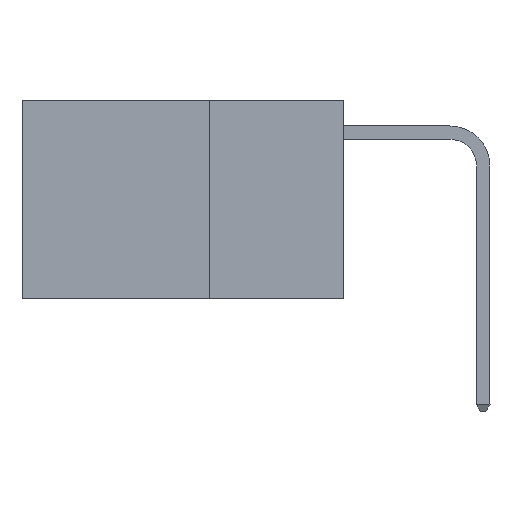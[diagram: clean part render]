
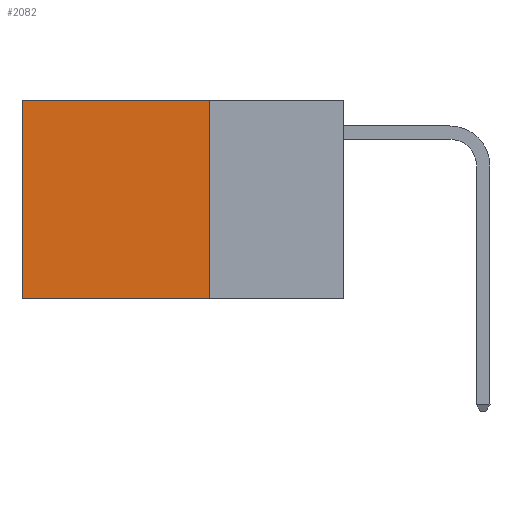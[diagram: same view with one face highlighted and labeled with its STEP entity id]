
A CAD part, left-side view. The second image highlights one B-rep face of the part: STEP entity #2082.
In plain terms, the highlighted planar face has unit normal (-1, 0, 0).
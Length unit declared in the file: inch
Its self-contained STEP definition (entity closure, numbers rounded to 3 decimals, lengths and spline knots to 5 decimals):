
#605 = VERTEX_POINT ( 'NONE', #11744 ) ;
#836 = LINE ( 'NONE', #6273, #850 ) ;
#850 = VECTOR ( 'NONE', #6244, 39.37008 ) ;
#907 = DIRECTION ( 'NONE',  ( 0., 0., -1. ) ) ;
#923 = DIRECTION ( 'NONE',  ( 1., 0., 0. ) ) ;
#956 = PLANE ( 'NONE',  #11997 ) ;
#990 = CARTESIAN_POINT ( 'NONE',  ( 0.2625, 0.25, 0. ) ) ;
#2082 = ADVANCED_FACE ( 'NONE', ( #12738 ), #956, .F. ) ;
#2351 = VECTOR ( 'NONE', #11156, 39.37008 ) ;
#2353 = LINE ( 'NONE', #11187, #2351 ) ;
#2980 = EDGE_CURVE ( 'NONE', #9294, #10404, #9688, .T. ) ;
#4439 = ORIENTED_EDGE ( 'NONE', *, *, #9593, .T. ) ;
#4444 = ORIENTED_EDGE ( 'NONE', *, *, #9288, .F. ) ;
#4579 = ORIENTED_EDGE ( 'NONE', *, *, #2980, .F. ) ;
#4589 = ORIENTED_EDGE ( 'NONE', *, *, #5637, .T. ) ;
#4631 = CARTESIAN_POINT ( 'NONE',  ( 0.2625, 0.25, -0.37 ) ) ;
#4886 = CARTESIAN_POINT ( 'NONE',  ( 0.2625, 0.6, -0.37 ) ) ;
#5637 = EDGE_CURVE ( 'NONE', #9294, #605, #5860, .T. ) ;
#5749 = VECTOR ( 'NONE', #7642, 39.37008 ) ;
#5860 = LINE ( 'NONE', #7692, #5749 ) ;
#6024 = VERTEX_POINT ( 'NONE', #4886 ) ;
#6244 = DIRECTION ( 'NONE',  ( 0., 0., -1. ) ) ;
#6273 = CARTESIAN_POINT ( 'NONE',  ( 0.2625, 0.6, 0. ) ) ;
#7642 = DIRECTION ( 'NONE',  ( 0., 1., 0. ) ) ;
#7692 = CARTESIAN_POINT ( 'NONE',  ( 0.2625, 0.25, 0. ) ) ;
#9288 = EDGE_CURVE ( 'NONE', #10404, #6024, #2353, .T. ) ;
#9294 = VERTEX_POINT ( 'NONE', #11041 ) ;
#9436 = VECTOR ( 'NONE', #10744, 39.37008 ) ;
#9593 = EDGE_CURVE ( 'NONE', #605, #6024, #836, .T. ) ;
#9688 = LINE ( 'NONE', #10834, #9436 ) ;
#10404 = VERTEX_POINT ( 'NONE', #4631 ) ;
#10744 = DIRECTION ( 'NONE',  ( 0., 0., -1. ) ) ;
#10834 = CARTESIAN_POINT ( 'NONE',  ( 0.2625, 0.25, 0. ) ) ;
#11041 = CARTESIAN_POINT ( 'NONE',  ( 0.2625, 0.25, 0. ) ) ;
#11156 = DIRECTION ( 'NONE',  ( 0., 1., 0. ) ) ;
#11187 = CARTESIAN_POINT ( 'NONE',  ( 0.2625, 0.25, -0.37 ) ) ;
#11744 = CARTESIAN_POINT ( 'NONE',  ( 0.2625, 0.6, 0. ) ) ;
#11820 = EDGE_LOOP ( 'NONE', ( #4439, #4444, #4579, #4589 ) ) ;
#11997 = AXIS2_PLACEMENT_3D ( 'NONE', #990, #923, #907 ) ;
#12738 = FACE_OUTER_BOUND ( 'NONE', #11820, .T. ) ;
